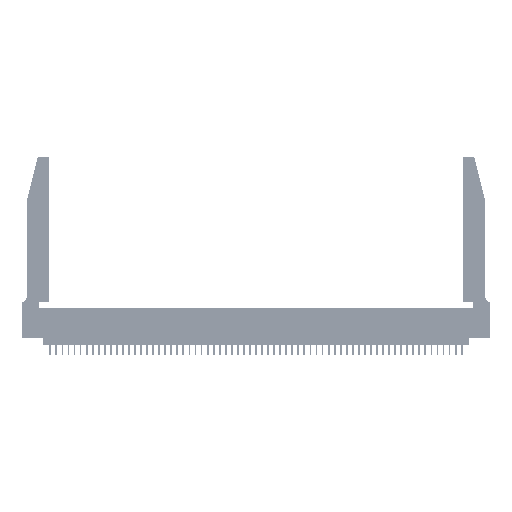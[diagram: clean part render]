
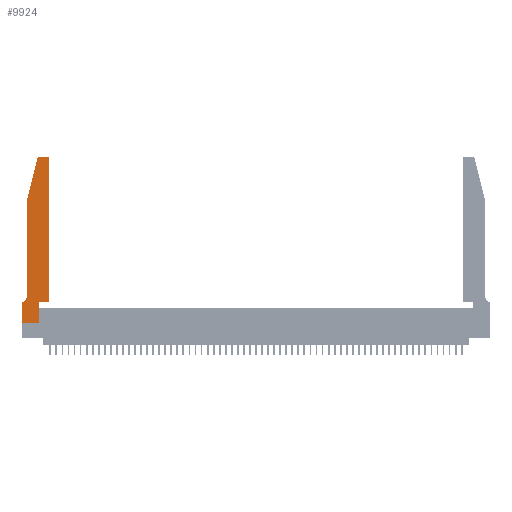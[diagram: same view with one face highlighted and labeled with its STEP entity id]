
A CAD part, top view. The second image highlights one B-rep face of the part: STEP entity #9924.
In plain terms, the highlighted planar face has unit normal (0, 0, 1).
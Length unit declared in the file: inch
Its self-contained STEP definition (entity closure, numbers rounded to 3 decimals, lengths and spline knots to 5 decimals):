
#347 = PLANE ( 'NONE',  #17102 ) ;
#645 = CARTESIAN_POINT ( 'NONE',  ( 0.284, 2.75, 0.37 ) ) ;
#715 = DIRECTION ( 'NONE',  ( 0., 0., 1. ) ) ;
#1723 = VERTEX_POINT ( 'NONE', #25264 ) ;
#3182 = DIRECTION ( 'NONE',  ( 1., 0., 0. ) ) ;
#3479 = LINE ( 'NONE', #6820, #45068 ) ;
#3818 = EDGE_CURVE ( 'NONE', #53824, #19532, #17944, .T. ) ;
#3920 = CARTESIAN_POINT ( 'NONE',  ( 0.0755, 2., 0.37 ) ) ;
#6791 = CARTESIAN_POINT ( 'NONE',  ( 0.2865, 0., 0.37 ) ) ;
#6820 = CARTESIAN_POINT ( 'NONE',  ( 0.0755, 2., 0.37 ) ) ;
#7407 = VECTOR ( 'NONE', #33731, 39.37008 ) ;
#7931 = ORIENTED_EDGE ( 'NONE', *, *, #44240, .T. ) ;
#8283 = DIRECTION ( 'NONE',  ( -0.239, -0.971, 0. ) ) ;
#8357 = CARTESIAN_POINT ( 'NONE',  ( 0.4505, 2.72, 0.37 ) ) ;
#8484 = CARTESIAN_POINT ( 'NONE',  ( 0.0755, 2., 0.37 ) ) ;
#8903 = ORIENTED_EDGE ( 'NONE', *, *, #31795, .T. ) ;
#8985 = ORIENTED_EDGE ( 'NONE', *, *, #35079, .T. ) ;
#9387 = AXIS2_PLACEMENT_3D ( 'NONE', #30465, #26523, #39279 ) ;
#9924 = ADVANCED_FACE ( 'NONE', ( #20431 ), #347, .T. ) ;
#10011 = VERTEX_POINT ( 'NONE', #52847 ) ;
#10425 = ORIENTED_EDGE ( 'NONE', *, *, #48695, .T. ) ;
#10514 = DIRECTION ( 'NONE',  ( 1., 0., 0. ) ) ;
#10959 = VERTEX_POINT ( 'NONE', #11281 ) ;
#11131 = DIRECTION ( 'NONE',  ( 0., -1., 0. ) ) ;
#11281 = CARTESIAN_POINT ( 'NONE',  ( 0.4505, 0.35, 0.37 ) ) ;
#12036 = DIRECTION ( 'NONE',  ( 0., -1., 0. ) ) ;
#13587 = VECTOR ( 'NONE', #8283, 39.37008 ) ;
#13619 = DIRECTION ( 'NONE',  ( 1., 0., 0. ) ) ;
#13939 = VERTEX_POINT ( 'NONE', #28808 ) ;
#14289 = ORIENTED_EDGE ( 'NONE', *, *, #27967, .T. ) ;
#14477 = ORIENTED_EDGE ( 'NONE', *, *, #3818, .T. ) ;
#14717 = ORIENTED_EDGE ( 'NONE', *, *, #49996, .T. ) ;
#15982 = CARTESIAN_POINT ( 'NONE',  ( 0., 0., 0.37 ) ) ;
#16567 = ORIENTED_EDGE ( 'NONE', *, *, #42772, .T. ) ;
#17102 = AXIS2_PLACEMENT_3D ( 'NONE', #51741, #715, #13619 ) ;
#17944 = CIRCLE ( 'NONE', #48920, 0.03 ) ;
#18158 = CIRCLE ( 'NONE', #9387, 0.07 ) ;
#18337 = CARTESIAN_POINT ( 'NONE',  ( 0.284, 2.72, 0.37 ) ) ;
#18649 = VECTOR ( 'NONE', #41840, 39.37008 ) ;
#19223 = LINE ( 'NONE', #36439, #48778 ) ;
#19532 = VERTEX_POINT ( 'NONE', #49628 ) ;
#20431 = FACE_OUTER_BOUND ( 'NONE', #34101, .T. ) ;
#21031 = VERTEX_POINT ( 'NONE', #8357 ) ;
#21243 = LINE ( 'NONE', #54422, #29325 ) ;
#22790 = ORIENTED_EDGE ( 'NONE', *, *, #37201, .T. ) ;
#23020 = LINE ( 'NONE', #15982, #33107 ) ;
#23253 = CARTESIAN_POINT ( 'NONE',  ( 0., 0., 0.37 ) ) ;
#23268 = CARTESIAN_POINT ( 'NONE',  ( 0.4505, 0.35, 0.37 ) ) ;
#23310 = CIRCLE ( 'NONE', #30777, 0.03 ) ;
#23776 = VERTEX_POINT ( 'NONE', #3920 ) ;
#24614 = VERTEX_POINT ( 'NONE', #44535 ) ;
#25264 = CARTESIAN_POINT ( 'NONE',  ( 0.4205, 2.75, 0.37 ) ) ;
#26523 = DIRECTION ( 'NONE',  ( 0., 0., -1. ) ) ;
#26598 = LINE ( 'NONE', #23268, #55421 ) ;
#27967 = EDGE_CURVE ( 'NONE', #21031, #1723, #23310, .T. ) ;
#28808 = CARTESIAN_POINT ( 'NONE',  ( 0.0055, 0.35, 0.37 ) ) ;
#29220 = EDGE_CURVE ( 'NONE', #1723, #53824, #21243, .T. ) ;
#29325 = VECTOR ( 'NONE', #49939, 39.37008 ) ;
#30465 = CARTESIAN_POINT ( 'NONE',  ( 0.0055, 0.42, 0.37 ) ) ;
#30777 = AXIS2_PLACEMENT_3D ( 'NONE', #42189, #37510, #3182 ) ;
#31795 = EDGE_CURVE ( 'NONE', #23776, #24614, #3479, .T. ) ;
#32326 = DIRECTION ( 'NONE',  ( 0., 1., 0. ) ) ;
#33107 = VECTOR ( 'NONE', #12036, 39.37008 ) ;
#33579 = EDGE_CURVE ( 'NONE', #10011, #10959, #26598, .T. ) ;
#33731 = DIRECTION ( 'NONE',  ( 0., 1., 0. ) ) ;
#33917 = CARTESIAN_POINT ( 'NONE',  ( 0.2865, 0.35, 0.37 ) ) ;
#34101 = EDGE_LOOP ( 'NONE', ( #48483, #14477, #8985, #8903, #7931, #54431, #16567, #10425, #22790, #54883, #14717, #14289 ) ) ;
#35035 = DIRECTION ( 'NONE',  ( 1., 0., 0. ) ) ;
#35079 = EDGE_CURVE ( 'NONE', #19532, #23776, #41809, .T. ) ;
#35844 = DIRECTION ( 'NONE',  ( 1., 0., 0. ) ) ;
#36439 = CARTESIAN_POINT ( 'NONE',  ( 0.4505, 0.35, 0.37 ) ) ;
#37201 = EDGE_CURVE ( 'NONE', #47806, #10011, #44994, .T. ) ;
#37510 = DIRECTION ( 'NONE',  ( 0., 0., 1. ) ) ;
#39279 = DIRECTION ( 'NONE',  ( -1., 0., 0. ) ) ;
#40430 = EDGE_CURVE ( 'NONE', #13939, #51156, #42144, .T. ) ;
#40536 = CARTESIAN_POINT ( 'NONE',  ( 0.0755, 0.35, 0.37 ) ) ;
#41809 = LINE ( 'NONE', #8484, #13587 ) ;
#41840 = DIRECTION ( 'NONE',  ( -1., 0., 0. ) ) ;
#42144 = LINE ( 'NONE', #40536, #18649 ) ;
#42189 = CARTESIAN_POINT ( 'NONE',  ( 0.4205, 2.72, 0.37 ) ) ;
#42197 = VECTOR ( 'NONE', #35844, 39.37008 ) ;
#42696 = VERTEX_POINT ( 'NONE', #51046 ) ;
#42772 = EDGE_CURVE ( 'NONE', #51156, #42696, #23020, .T. ) ;
#44240 = EDGE_CURVE ( 'NONE', #24614, #13939, #18158, .T. ) ;
#44535 = CARTESIAN_POINT ( 'NONE',  ( 0.0755, 0.42, 0.37 ) ) ;
#44994 = LINE ( 'NONE', #33917, #7407 ) ;
#45068 = VECTOR ( 'NONE', #11131, 39.37008 ) ;
#47632 = CARTESIAN_POINT ( 'NONE',  ( 0., 0.35, 0.37 ) ) ;
#47806 = VERTEX_POINT ( 'NONE', #6791 ) ;
#48240 = LINE ( 'NONE', #23253, #42197 ) ;
#48483 = ORIENTED_EDGE ( 'NONE', *, *, #29220, .T. ) ;
#48695 = EDGE_CURVE ( 'NONE', #42696, #47806, #48240, .T. ) ;
#48778 = VECTOR ( 'NONE', #32326, 39.37008 ) ;
#48920 = AXIS2_PLACEMENT_3D ( 'NONE', #18337, #51912, #35035 ) ;
#49628 = CARTESIAN_POINT ( 'NONE',  ( 0.25487, 2.72718, 0.37 ) ) ;
#49939 = DIRECTION ( 'NONE',  ( -1., 0., 0. ) ) ;
#49996 = EDGE_CURVE ( 'NONE', #10959, #21031, #19223, .T. ) ;
#51046 = CARTESIAN_POINT ( 'NONE',  ( 0., 0., 0.37 ) ) ;
#51156 = VERTEX_POINT ( 'NONE', #47632 ) ;
#51741 = CARTESIAN_POINT ( 'NONE',  ( 0., 0.35, 0.37 ) ) ;
#51912 = DIRECTION ( 'NONE',  ( 0., 0., 1. ) ) ;
#52847 = CARTESIAN_POINT ( 'NONE',  ( 0.2865, 0.35, 0.37 ) ) ;
#53824 = VERTEX_POINT ( 'NONE', #645 ) ;
#54422 = CARTESIAN_POINT ( 'NONE',  ( 0.2605, 2.75, 0.37 ) ) ;
#54431 = ORIENTED_EDGE ( 'NONE', *, *, #40430, .T. ) ;
#54883 = ORIENTED_EDGE ( 'NONE', *, *, #33579, .T. ) ;
#55421 = VECTOR ( 'NONE', #10514, 39.37008 ) ;
